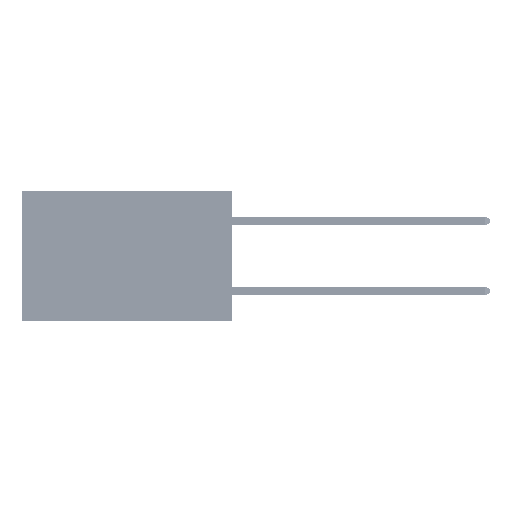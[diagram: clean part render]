
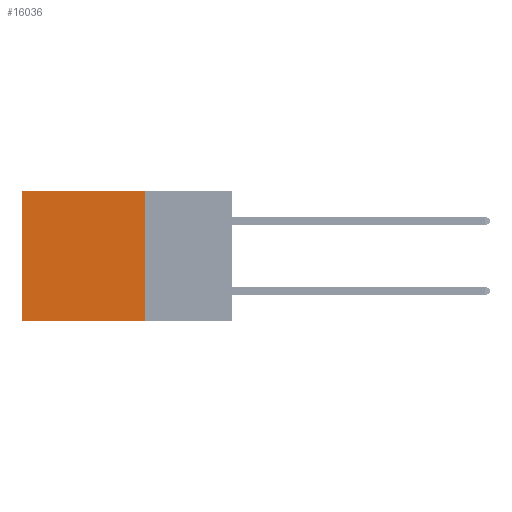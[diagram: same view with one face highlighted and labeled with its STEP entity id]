
A CAD part, left-side view. The second image highlights one B-rep face of the part: STEP entity #16036.
In plain terms, the highlighted planar face has unit normal (-1, 0, 0).
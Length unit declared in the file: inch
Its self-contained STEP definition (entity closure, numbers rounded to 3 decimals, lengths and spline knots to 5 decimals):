
#516 = LINE ( 'NONE', #48956, #47837 ) ;
#1921 = ORIENTED_EDGE ( 'NONE', *, *, #23815, .T. ) ;
#4703 = DIRECTION ( 'NONE',  ( 0., 0., -1. ) ) ;
#5576 = FACE_OUTER_BOUND ( 'NONE', #31838, .T. ) ;
#6513 = ORIENTED_EDGE ( 'NONE', *, *, #43810, .T. ) ;
#7685 = VERTEX_POINT ( 'NONE', #17991 ) ;
#11794 = DIRECTION ( 'NONE',  ( 0., 1., 0. ) ) ;
#12331 = CARTESIAN_POINT ( 'NONE',  ( 0.2875, 0.25, 0. ) ) ;
#13362 = CARTESIAN_POINT ( 'NONE',  ( 0.2875, 0.25, 0. ) ) ;
#16036 = ADVANCED_FACE ( 'NONE', ( #5576 ), #42584, .F. ) ;
#17991 = CARTESIAN_POINT ( 'NONE',  ( 0.2875, 0.25, 0. ) ) ;
#18457 = CARTESIAN_POINT ( 'NONE',  ( 0.2875, 0.25, 0. ) ) ;
#18909 = VERTEX_POINT ( 'NONE', #35467 ) ;
#19806 = VERTEX_POINT ( 'NONE', #48317 ) ;
#20545 = LINE ( 'NONE', #12331, #30286 ) ;
#21205 = VECTOR ( 'NONE', #26948, 39.37008 ) ;
#21318 = LINE ( 'NONE', #48838, #39564 ) ;
#23030 = EDGE_CURVE ( 'NONE', #18909, #52663, #21318, .T. ) ;
#23815 = EDGE_CURVE ( 'NONE', #19806, #52663, #516, .T. ) ;
#25220 = ORIENTED_EDGE ( 'NONE', *, *, #29149, .F. ) ;
#26948 = DIRECTION ( 'NONE',  ( 0., 0., -1. ) ) ;
#28204 = DIRECTION ( 'NONE',  ( 0., 0., -1. ) ) ;
#29149 = EDGE_CURVE ( 'NONE', #7685, #18909, #44671, .T. ) ;
#30286 = VECTOR ( 'NONE', #11794, 39.37008 ) ;
#30962 = CARTESIAN_POINT ( 'NONE',  ( 0.2875, 0.6, -0.37 ) ) ;
#31838 = EDGE_LOOP ( 'NONE', ( #1921, #33296, #25220, #6513 ) ) ;
#33296 = ORIENTED_EDGE ( 'NONE', *, *, #23030, .F. ) ;
#35467 = CARTESIAN_POINT ( 'NONE',  ( 0.2875, 0.25, -0.37 ) ) ;
#39564 = VECTOR ( 'NONE', #44313, 39.37008 ) ;
#42584 = PLANE ( 'NONE',  #52847 ) ;
#43810 = EDGE_CURVE ( 'NONE', #7685, #19806, #20545, .T. ) ;
#44313 = DIRECTION ( 'NONE',  ( 0., 1., 0. ) ) ;
#44671 = LINE ( 'NONE', #18457, #21205 ) ;
#46583 = DIRECTION ( 'NONE',  ( 1., 0., 0. ) ) ;
#47837 = VECTOR ( 'NONE', #28204, 39.37008 ) ;
#48317 = CARTESIAN_POINT ( 'NONE',  ( 0.2875, 0.6, 0. ) ) ;
#48838 = CARTESIAN_POINT ( 'NONE',  ( 0.2875, 0.25, -0.37 ) ) ;
#48956 = CARTESIAN_POINT ( 'NONE',  ( 0.2875, 0.6, 0. ) ) ;
#52663 = VERTEX_POINT ( 'NONE', #30962 ) ;
#52847 = AXIS2_PLACEMENT_3D ( 'NONE', #13362, #46583, #4703 ) ;
